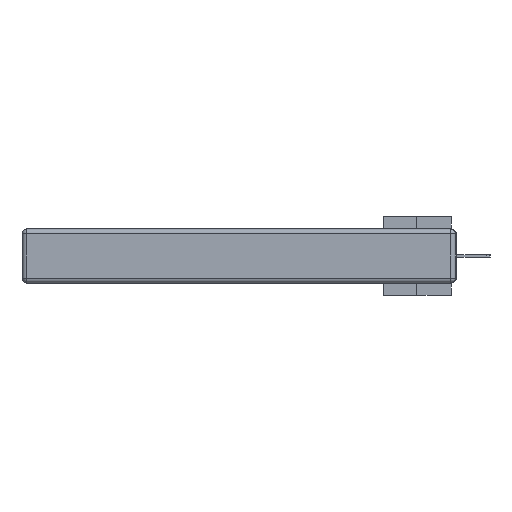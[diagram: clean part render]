
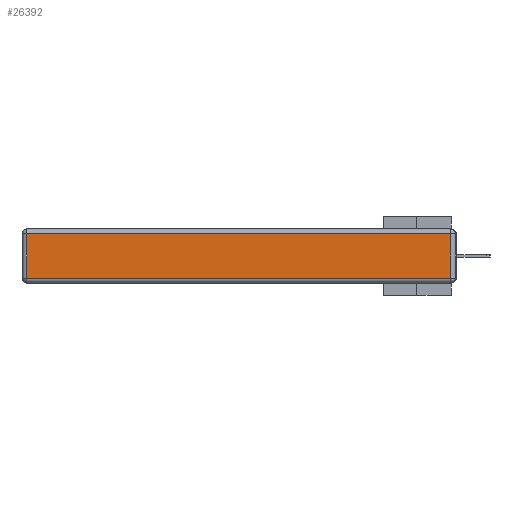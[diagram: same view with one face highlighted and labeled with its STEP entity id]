
A CAD part, left-side view. The second image highlights one B-rep face of the part: STEP entity #26392.
In plain terms, the highlighted planar face has unit normal (-1, 0, 0).
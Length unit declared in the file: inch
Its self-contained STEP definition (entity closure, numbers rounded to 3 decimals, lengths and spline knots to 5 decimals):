
#99 = ORIENTED_EDGE ( 'NONE', *, *, #17627, .T. ) ;
#177 = VECTOR ( 'NONE', #10495, 39.37008 ) ;
#2214 = VERTEX_POINT ( 'NONE', #32271 ) ;
#2416 = DIRECTION ( 'NONE',  ( -1., 0., 0. ) ) ;
#3574 = CARTESIAN_POINT ( 'NONE',  ( 0., 2.75, -0.03 ) ) ;
#4554 = ORIENTED_EDGE ( 'NONE', *, *, #19346, .T. ) ;
#7314 = CARTESIAN_POINT ( 'NONE',  ( 0., 2.72, -0.313 ) ) ;
#7914 = LINE ( 'NONE', #23383, #29080 ) ;
#8301 = DIRECTION ( 'NONE',  ( 0., 1., 0. ) ) ;
#8561 = DIRECTION ( 'NONE',  ( 0., -1., 0. ) ) ;
#10029 = DIRECTION ( 'NONE',  ( 0., 0., -1. ) ) ;
#10495 = DIRECTION ( 'NONE',  ( 0., 0., 1. ) ) ;
#13997 = LINE ( 'NONE', #24535, #177 ) ;
#16836 = VECTOR ( 'NONE', #8301, 39.37008 ) ;
#17627 = EDGE_CURVE ( 'NONE', #30825, #26374, #7914, .T. ) ;
#18277 = EDGE_CURVE ( 'NONE', #26374, #24851, #19107, .T. ) ;
#19107 = LINE ( 'NONE', #32592, #20149 ) ;
#19346 = EDGE_CURVE ( 'NONE', #2214, #30825, #32863, .T. ) ;
#19951 = ORIENTED_EDGE ( 'NONE', *, *, #34245, .T. ) ;
#20149 = VECTOR ( 'NONE', #8561, 39.37008 ) ;
#21171 = FACE_OUTER_BOUND ( 'NONE', #29528, .T. ) ;
#22666 = AXIS2_PLACEMENT_3D ( 'NONE', #26448, #2416, #29765 ) ;
#23383 = CARTESIAN_POINT ( 'NONE',  ( 0., 2.72, -0.343 ) ) ;
#24394 = CARTESIAN_POINT ( 'NONE',  ( 0., 2.72, -0.03 ) ) ;
#24535 = CARTESIAN_POINT ( 'NONE',  ( 0., 0.03, -0.343 ) ) ;
#24851 = VERTEX_POINT ( 'NONE', #26999 ) ;
#26374 = VERTEX_POINT ( 'NONE', #7314 ) ;
#26392 = ADVANCED_FACE ( 'NONE', ( #21171 ), #29427, .T. ) ;
#26448 = CARTESIAN_POINT ( 'NONE',  ( 0., 0., -0.343 ) ) ;
#26999 = CARTESIAN_POINT ( 'NONE',  ( 0., 0.03, -0.313 ) ) ;
#29080 = VECTOR ( 'NONE', #10029, 39.37008 ) ;
#29427 = PLANE ( 'NONE',  #22666 ) ;
#29528 = EDGE_LOOP ( 'NONE', ( #33580, #19951, #4554, #99 ) ) ;
#29765 = DIRECTION ( 'NONE',  ( 0., 0., 1. ) ) ;
#30825 = VERTEX_POINT ( 'NONE', #24394 ) ;
#32271 = CARTESIAN_POINT ( 'NONE',  ( 0., 0.03, -0.03 ) ) ;
#32592 = CARTESIAN_POINT ( 'NONE',  ( 0., 0., -0.313 ) ) ;
#32863 = LINE ( 'NONE', #3574, #16836 ) ;
#33580 = ORIENTED_EDGE ( 'NONE', *, *, #18277, .T. ) ;
#34245 = EDGE_CURVE ( 'NONE', #24851, #2214, #13997, .T. ) ;
